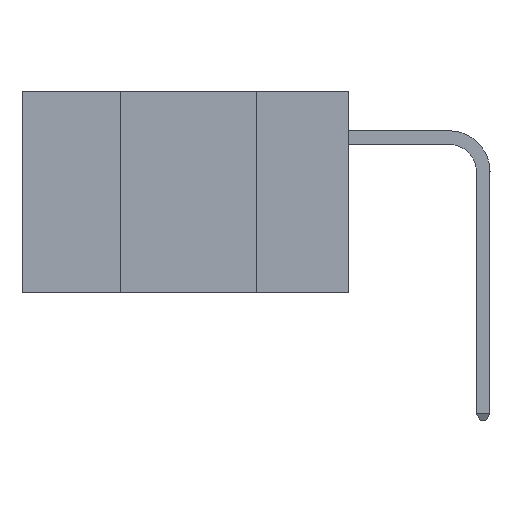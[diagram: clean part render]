
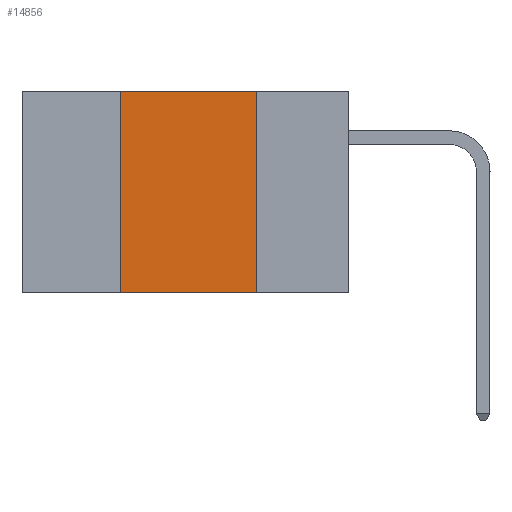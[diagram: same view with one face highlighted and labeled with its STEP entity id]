
A CAD part, left-side view. The second image highlights one B-rep face of the part: STEP entity #14856.
In plain terms, the highlighted planar face has unit normal (-1, 0, 0).
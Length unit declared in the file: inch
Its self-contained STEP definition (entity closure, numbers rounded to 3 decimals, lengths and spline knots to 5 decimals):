
#433 = PLANE ( 'NONE',  #1393 ) ;
#1393 = AXIS2_PLACEMENT_3D ( 'NONE', #1905, #11757, #3373 ) ;
#1472 = CARTESIAN_POINT ( 'NONE',  ( 0., 0.17, -0.37 ) ) ;
#1905 = CARTESIAN_POINT ( 'NONE',  ( 0., 0.6, 0. ) ) ;
#2186 = LINE ( 'NONE', #14231, #9212 ) ;
#2949 = LINE ( 'NONE', #10499, #17327 ) ;
#3256 = EDGE_CURVE ( 'NONE', #11335, #6324, #2186, .T. ) ;
#3373 = DIRECTION ( 'NONE',  ( 0., 0., -1. ) ) ;
#3831 = EDGE_LOOP ( 'NONE', ( #6041, #7133, #9056, #11270 ) ) ;
#4282 = VERTEX_POINT ( 'NONE', #8952 ) ;
#4613 = FACE_OUTER_BOUND ( 'NONE', #3831, .T. ) ;
#6041 = ORIENTED_EDGE ( 'NONE', *, *, #18143, .F. ) ;
#6324 = VERTEX_POINT ( 'NONE', #1472 ) ;
#6327 = DIRECTION ( 'NONE',  ( 0., -1., 0. ) ) ;
#7003 = VERTEX_POINT ( 'NONE', #14899 ) ;
#7133 = ORIENTED_EDGE ( 'NONE', *, *, #17272, .F. ) ;
#7914 = EDGE_CURVE ( 'NONE', #11335, #7003, #14829, .T. ) ;
#8460 = CARTESIAN_POINT ( 'NONE',  ( 0., 0.17, 0. ) ) ;
#8952 = CARTESIAN_POINT ( 'NONE',  ( 0., 0.17, 0. ) ) ;
#9056 = ORIENTED_EDGE ( 'NONE', *, *, #7914, .F. ) ;
#9212 = VECTOR ( 'NONE', #15584, 39.37008 ) ;
#10499 = CARTESIAN_POINT ( 'NONE',  ( 0., 0.6, 0. ) ) ;
#11110 = VECTOR ( 'NONE', #12675, 39.37008 ) ;
#11270 = ORIENTED_EDGE ( 'NONE', *, *, #3256, .T. ) ;
#11335 = VERTEX_POINT ( 'NONE', #14541 ) ;
#11757 = DIRECTION ( 'NONE',  ( 1., 0., 0. ) ) ;
#12675 = DIRECTION ( 'NONE',  ( 0., 0., 1. ) ) ;
#12722 = DIRECTION ( 'NONE',  ( 0., 0., -1. ) ) ;
#13227 = VECTOR ( 'NONE', #12722, 39.37008 ) ;
#14231 = CARTESIAN_POINT ( 'NONE',  ( 0., 0.6, -0.37 ) ) ;
#14541 = CARTESIAN_POINT ( 'NONE',  ( 0., 0.42, -0.37 ) ) ;
#14829 = LINE ( 'NONE', #16761, #11110 ) ;
#14856 = ADVANCED_FACE ( 'NONE', ( #4613 ), #433, .F. ) ;
#14899 = CARTESIAN_POINT ( 'NONE',  ( 0., 0.42, 0. ) ) ;
#15584 = DIRECTION ( 'NONE',  ( 0., -1., 0. ) ) ;
#16012 = LINE ( 'NONE', #8460, #13227 ) ;
#16761 = CARTESIAN_POINT ( 'NONE',  ( 0., 0.42, 0. ) ) ;
#17272 = EDGE_CURVE ( 'NONE', #7003, #4282, #2949, .T. ) ;
#17327 = VECTOR ( 'NONE', #6327, 39.37008 ) ;
#18143 = EDGE_CURVE ( 'NONE', #4282, #6324, #16012, .T. ) ;
